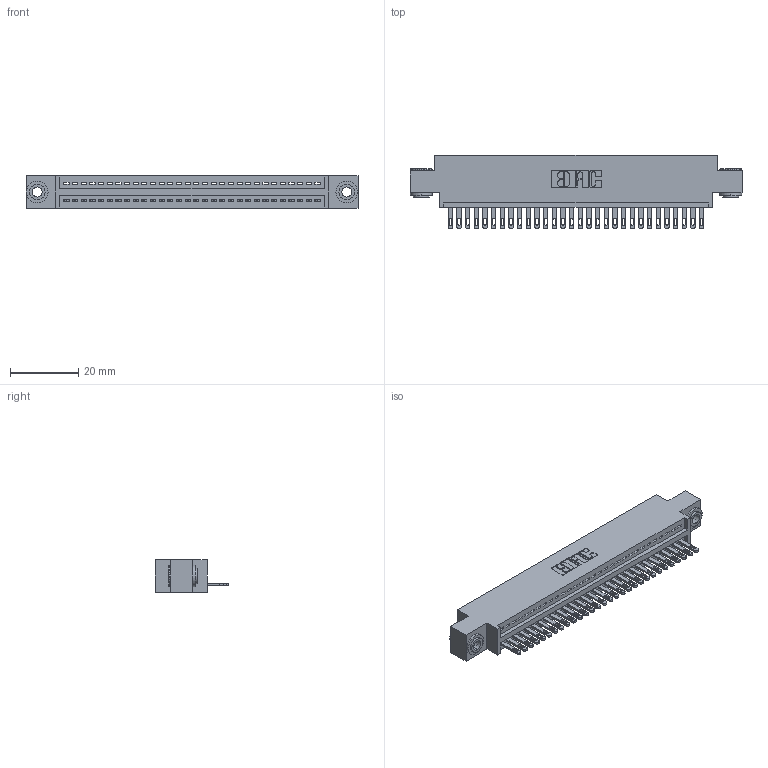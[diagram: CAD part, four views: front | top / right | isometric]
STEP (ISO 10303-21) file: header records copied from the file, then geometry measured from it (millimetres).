
FILE_DESCRIPTION (( 'STEP AP203' ), '1' );
FILE_NAME ('895-030-500-603.STEP', '2020-09-25T17:51:16', ( '' ), ( '' ), 'SwSTEP 2.0', 'SolidWorks 2020', '' );
FILE_SCHEMA (( 'CONFIG_CONTROL_DESIGN' ));
Length unit declared in the file: inch
Products named in the file (4): 845 Part_0.170 Offset - 0.156 Dia-TH; 345-250-002_345-250-002-102; 345-292-001_345-293-100; 895-030-500-603
Assembly tree (33 placements, depth 2):
  895-030-500-603
    845 Part_0.170 Offset - 0.156 Dia-TH
    345-292-001_345-293-100  x30
    345-250-002_345-250-002-102  x2
Bounding box: 97.41 x 21.51 x 9.4 mm (x, y, z)
Volume: 9078.3 mm3; surface area: 12309.5 mm2
Topology: 33 solids, 33 shells, 1788 faces, 5469 edges, 3642 vertices
Faces by surface type: plane 1114, cylinder 666, cone 8
Entity records: 24906 total; most frequent: CARTESIAN_POINT 4293, ORIENTED_EDGE 4250, DIRECTION 3799, EDGE_CURVE 2125, VECTOR 1845, LINE 1845, VERTEX_POINT 1414, AXIS2_PLACEMENT_3D 977
